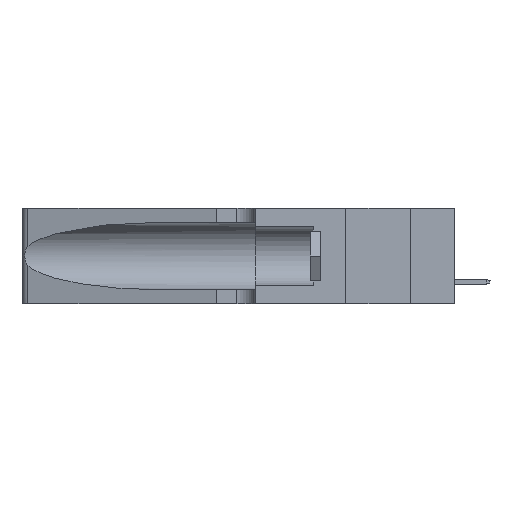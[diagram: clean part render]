
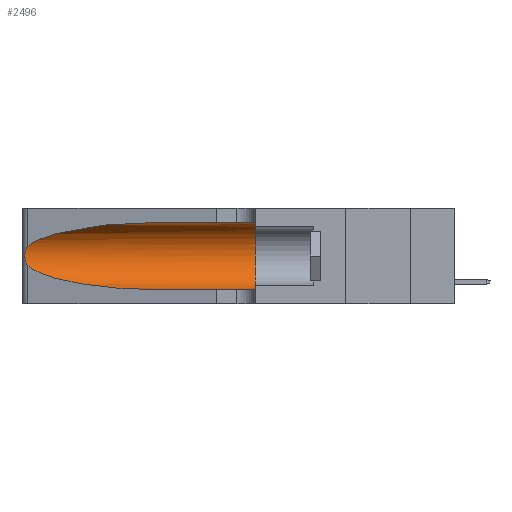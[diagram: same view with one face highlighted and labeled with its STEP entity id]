
A CAD part, left-side view. The second image highlights one B-rep face of the part: STEP entity #2496.
In plain terms, the highlighted cylindrical face has radius 3.308 mm (diameter 6.617 mm), a partial arc.
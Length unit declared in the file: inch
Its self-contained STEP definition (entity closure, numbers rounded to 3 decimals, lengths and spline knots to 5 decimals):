
#1455 = CARTESIAN_POINT ( 'NONE',  ( 0.25487, 1.22718, 0.22369 ) ) ;
#1520 = CARTESIAN_POINT ( 'NONE',  ( 0.1305, 0.72297, 0.31525 ) ) ;
#1654 = VERTEX_POINT ( 'NONE', #15782 ) ;
#1745 = CARTESIAN_POINT ( 'NONE',  ( 0.1305, 0.35, 0.31525 ) ) ;
#2401 = DIRECTION ( 'NONE',  ( 0., -1., 0. ) ) ;
#2496 = ADVANCED_FACE ( 'NONE', ( #11743 ), #28139, .F. ) ;
#2949 = DIRECTION ( 'NONE',  ( 0., 0., 1. ) ) ;
#3404 = CARTESIAN_POINT ( 'NONE',  ( 0.1305, 1.61858, 0.31525 ) ) ;
#3441 = CARTESIAN_POINT ( 'NONE',  ( 0.25487, 1.22718, 0.14631 ) ) ;
#3694 = CARTESIAN_POINT ( 'NONE',  ( 0.2373, 1.15595, 0.08982 ) ) ;
#3715 = CARTESIAN_POINT ( 'NONE',  ( 0.18966, 0.96281, 0.31525 ) ) ;
#3849 = CARTESIAN_POINT ( 'NONE',  ( 0.25487, 1.22718, 0.14631 ) ) ;
#4263 = CARTESIAN_POINT ( 'NONE',  ( 0.26075, 1.23896, 0.178 ) ) ;
#5353 = AXIS2_PLACEMENT_3D ( 'NONE', #25787, #27989, #19096 ) ;
#5735 = CARTESIAN_POINT ( 'NONE',  ( 0.1305, 0.72297, 0.05475 ) ) ;
#5906 = DIRECTION ( 'NONE',  ( 0., -1., 0. ) ) ;
#6160 = CARTESIAN_POINT ( 'NONE',  ( 0.25555, 1.22994, 0.2215 ) ) ;
#6307 = CARTESIAN_POINT ( 'NONE',  ( 0.26075, 1.23896, 0.19203 ) ) ;
#6759 = CARTESIAN_POINT ( 'NONE',  ( 0.25854, 1.2359, 0.20912 ) ) ;
#7039 = EDGE_CURVE ( 'NONE', #1654, #11394, #7315, .T. ) ;
#7205 = CARTESIAN_POINT ( 'NONE',  ( 0.1305, 0.72297, 0.05475 ) ) ;
#7315 = B_SPLINE_CURVE_WITH_KNOTS ( 'NONE', 3,
 ( #1455, #6160, #13354, #8807, #6759, #11014, #6307, #4263, #30521, #11466, #25362, #13507, #9120, #27864 ),
 .UNSPECIFIED., .F., .F.,
 ( 4, 2, 2, 2, 2, 2, 4 ),
 ( 0., 0.00027, 0.00053, 0.00107, 0.0016, 0.00187, 0.00214 ),
 .UNSPECIFIED. ) ;
#8807 = CARTESIAN_POINT ( 'NONE',  ( 0.25787, 1.23484, 0.2124 ) ) ;
#8989 = AXIS2_PLACEMENT_3D ( 'NONE', #12192, #14377, #2949 ) ;
#9120 = CARTESIAN_POINT ( 'NONE',  ( 0.25555, 1.22993, 0.14849 ) ) ;
#9289 = CARTESIAN_POINT ( 'NONE',  ( 0.1305, 1.61858, 0.05475 ) ) ;
#9912 = VERTEX_POINT ( 'NONE', #7205 ) ;
#11014 = CARTESIAN_POINT ( 'NONE',  ( 0.26018, 1.23835, 0.19895 ) ) ;
#11067 = VERTEX_POINT ( 'NONE', #1745 ) ;
#11394 = VERTEX_POINT ( 'NONE', #3441 ) ;
#11466 = CARTESIAN_POINT ( 'NONE',  ( 0.25856, 1.23593, 0.16098 ) ) ;
#11743 = FACE_OUTER_BOUND ( 'NONE', #23412, .T. ) ;
#11783 = EDGE_CURVE ( 'NONE', #14430, #11067, #13245, .T. ) ;
#12192 = CARTESIAN_POINT ( 'NONE',  ( 0.1305, 0.35, 0.185 ) ) ;
#12921 = EDGE_CURVE ( 'NONE', #11067, #16568, #22427, .T. ) ;
#13245 = LINE ( 'NONE', #3404, #21884 ) ;
#13354 = CARTESIAN_POINT ( 'NONE',  ( 0.25639, 1.23184, 0.21858 ) ) ;
#13507 = CARTESIAN_POINT ( 'NONE',  ( 0.25639, 1.23186, 0.15144 ) ) ;
#14377 = DIRECTION ( 'NONE',  ( 0., 1., 0. ) ) ;
#14430 = VERTEX_POINT ( 'NONE', #18498 ) ;
#15782 = CARTESIAN_POINT ( 'NONE',  ( 0.25487, 1.22718, 0.22369 ) ) ;
#15876 = ORIENTED_EDGE ( 'NONE', *, *, #12921, .F. ) ;
#16568 = VERTEX_POINT ( 'NONE', #21518 ) ;
#16794 = EDGE_CURVE ( 'NONE', #11394, #9912, #24857, .T. ) ;
#18111 = CARTESIAN_POINT ( 'NONE',  ( 0.25487, 1.22718, 0.22369 ) ) ;
#18439 = ORIENTED_EDGE ( 'NONE', *, *, #11783, .F. ) ;
#18498 = CARTESIAN_POINT ( 'NONE',  ( 0.1305, 0.72297, 0.31525 ) ) ;
#19096 = DIRECTION ( 'NONE',  ( 0., 0., -1. ) ) ;
#19484 =( BOUNDED_CURVE ( )  B_SPLINE_CURVE ( 3, ( #1520, #3715, #25264, #18111 ),
 .UNSPECIFIED., .F., .T. ) 
 B_SPLINE_CURVE_WITH_KNOTS ( ( 4, 4 ),
 ( 1.5708, 2.84003 ),
 .UNSPECIFIED. ) 
 CURVE ( )  GEOMETRIC_REPRESENTATION_ITEM ( )  RATIONAL_B_SPLINE_CURVE ( ( 1., 0.87, 0.87, 1. ) ) 
 REPRESENTATION_ITEM ( '' )  );
#20088 = ORIENTED_EDGE ( 'NONE', *, *, #7039, .T. ) ;
#21518 = CARTESIAN_POINT ( 'NONE',  ( 0.1305, 0.35, 0.05475 ) ) ;
#21884 = VECTOR ( 'NONE', #5906, 39.37008 ) ;
#22129 = EDGE_CURVE ( 'NONE', #9912, #16568, #28812, .T. ) ;
#22351 = ORIENTED_EDGE ( 'NONE', *, *, #28838, .T. ) ;
#22427 = CIRCLE ( 'NONE', #8989, 0.13025 ) ;
#22728 = CARTESIAN_POINT ( 'NONE',  ( 0.18966, 0.96281, 0.05475 ) ) ;
#23412 = EDGE_LOOP ( 'NONE', ( #22351, #20088, #26029, #26534, #15876, #18439 ) ) ;
#24284 = VECTOR ( 'NONE', #2401, 39.37008 ) ;
#24857 =( BOUNDED_CURVE ( )  B_SPLINE_CURVE ( 3, ( #3849, #3694, #22728, #5735 ),
 .UNSPECIFIED., .F., .F. ) 
 B_SPLINE_CURVE_WITH_KNOTS ( ( 4, 4 ),
 ( 3.44316, 4.71239 ),
 .UNSPECIFIED. ) 
 CURVE ( )  GEOMETRIC_REPRESENTATION_ITEM ( )  RATIONAL_B_SPLINE_CURVE ( ( 1., 0.87, 0.87, 1. ) ) 
 REPRESENTATION_ITEM ( '' )  );
#25264 = CARTESIAN_POINT ( 'NONE',  ( 0.2373, 1.15595, 0.28018 ) ) ;
#25362 = CARTESIAN_POINT ( 'NONE',  ( 0.25789, 1.23486, 0.15765 ) ) ;
#25787 = CARTESIAN_POINT ( 'NONE',  ( 0.1305, 1.61858, 0.185 ) ) ;
#26029 = ORIENTED_EDGE ( 'NONE', *, *, #16794, .T. ) ;
#26534 = ORIENTED_EDGE ( 'NONE', *, *, #22129, .T. ) ;
#27864 = CARTESIAN_POINT ( 'NONE',  ( 0.25487, 1.22718, 0.14631 ) ) ;
#27989 = DIRECTION ( 'NONE',  ( 0., -1., 0. ) ) ;
#28139 = CYLINDRICAL_SURFACE ( 'NONE', #5353, 0.13025 ) ;
#28812 = LINE ( 'NONE', #9289, #24284 ) ;
#28838 = EDGE_CURVE ( 'NONE', #14430, #1654, #19484, .T. ) ;
#30521 = CARTESIAN_POINT ( 'NONE',  ( 0.26017, 1.23833, 0.17102 ) ) ;
